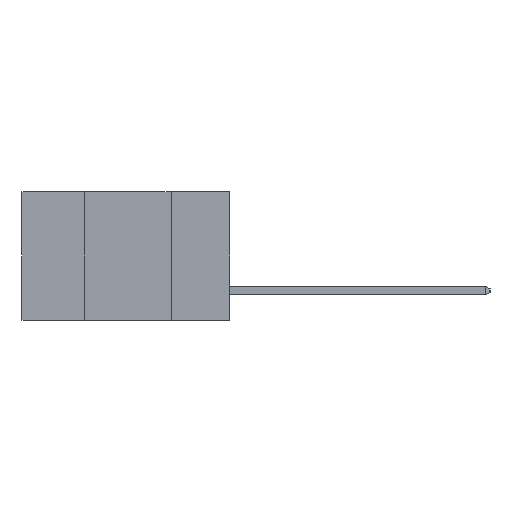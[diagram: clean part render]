
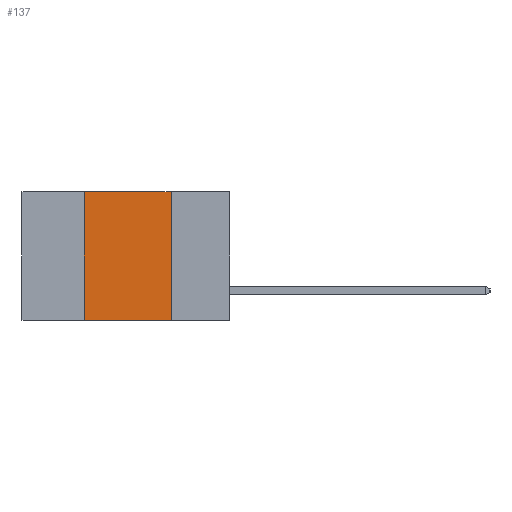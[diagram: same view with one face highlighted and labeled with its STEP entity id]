
A CAD part, left-side view. The second image highlights one B-rep face of the part: STEP entity #137.
In plain terms, the highlighted planar face has unit normal (-1, 0, 0).
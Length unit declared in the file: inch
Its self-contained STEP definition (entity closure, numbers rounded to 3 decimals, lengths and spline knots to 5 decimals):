
#137 = ADVANCED_FACE ( 'NONE', ( #8138 ), #2959, .F. ) ;
#468 = EDGE_CURVE ( 'NONE', #1625, #4209, #3726, .T. ) ;
#494 = CARTESIAN_POINT ( 'NONE',  ( 0., 0.6, 0. ) ) ;
#942 = EDGE_CURVE ( 'NONE', #2031, #1625, #5161, .T. ) ;
#1067 = DIRECTION ( 'NONE',  ( 0., 0., -1. ) ) ;
#1456 = EDGE_CURVE ( 'NONE', #2031, #2685, #4705, .T. ) ;
#1484 = CARTESIAN_POINT ( 'NONE',  ( 0., 0.17, 0. ) ) ;
#1485 = EDGE_LOOP ( 'NONE', ( #3357, #2622, #8216, #2398 ) ) ;
#1625 = VERTEX_POINT ( 'NONE', #4397 ) ;
#2031 = VERTEX_POINT ( 'NONE', #6718 ) ;
#2304 = CARTESIAN_POINT ( 'NONE',  ( 0., 0.42, -0.37 ) ) ;
#2361 = EDGE_CURVE ( 'NONE', #4209, #2685, #3236, .T. ) ;
#2398 = ORIENTED_EDGE ( 'NONE', *, *, #1456, .T. ) ;
#2622 = ORIENTED_EDGE ( 'NONE', *, *, #468, .F. ) ;
#2685 = VERTEX_POINT ( 'NONE', #5036 ) ;
#2834 = DIRECTION ( 'NONE',  ( 0., 0., 1. ) ) ;
#2921 = CARTESIAN_POINT ( 'NONE',  ( 0., 0.17, -0.37 ) ) ;
#2959 = PLANE ( 'NONE',  #7972 ) ;
#3236 = LINE ( 'NONE', #2921, #8090 ) ;
#3357 = ORIENTED_EDGE ( 'NONE', *, *, #2361, .F. ) ;
#3726 = LINE ( 'NONE', #494, #7020 ) ;
#4209 = VERTEX_POINT ( 'NONE', #1484 ) ;
#4397 = CARTESIAN_POINT ( 'NONE',  ( 0., 0.42, 0. ) ) ;
#4705 = LINE ( 'NONE', #8088, #8112 ) ;
#4781 = DIRECTION ( 'NONE',  ( 0., 0., -1. ) ) ;
#5036 = CARTESIAN_POINT ( 'NONE',  ( 0., 0.17, -0.37 ) ) ;
#5161 = LINE ( 'NONE', #2304, #6780 ) ;
#5864 = DIRECTION ( 'NONE',  ( 0., -1., 0. ) ) ;
#6258 = DIRECTION ( 'NONE',  ( 1., 0., 0. ) ) ;
#6291 = DIRECTION ( 'NONE',  ( 0., -1., 0. ) ) ;
#6718 = CARTESIAN_POINT ( 'NONE',  ( 0., 0.42, -0.37 ) ) ;
#6780 = VECTOR ( 'NONE', #2834, 39.37008 ) ;
#7020 = VECTOR ( 'NONE', #6291, 39.37008 ) ;
#7125 = CARTESIAN_POINT ( 'NONE',  ( 0., 0.6, 0. ) ) ;
#7972 = AXIS2_PLACEMENT_3D ( 'NONE', #7125, #6258, #1067 ) ;
#8088 = CARTESIAN_POINT ( 'NONE',  ( 0., 0.6, -0.37 ) ) ;
#8090 = VECTOR ( 'NONE', #4781, 39.37008 ) ;
#8112 = VECTOR ( 'NONE', #5864, 39.37008 ) ;
#8138 = FACE_OUTER_BOUND ( 'NONE', #1485, .T. ) ;
#8216 = ORIENTED_EDGE ( 'NONE', *, *, #942, .F. ) ;
